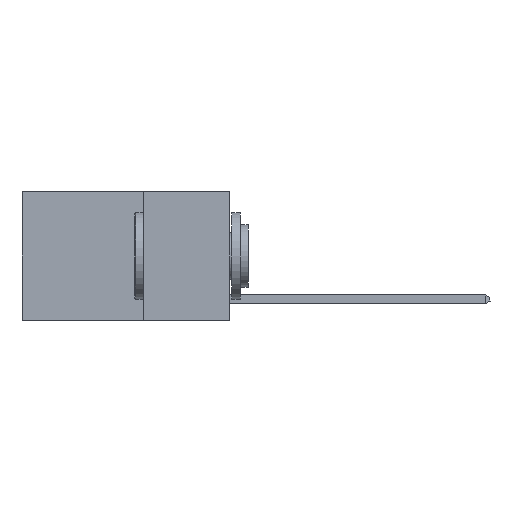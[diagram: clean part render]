
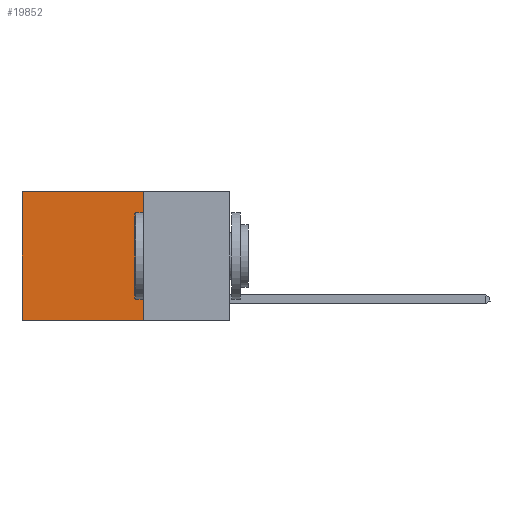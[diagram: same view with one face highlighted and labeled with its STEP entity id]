
A CAD part, left-side view. The second image highlights one B-rep face of the part: STEP entity #19852.
In plain terms, the highlighted planar face has unit normal (-1, 0, 0).
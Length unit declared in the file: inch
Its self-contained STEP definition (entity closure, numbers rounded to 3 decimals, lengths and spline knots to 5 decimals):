
#639 = AXIS2_PLACEMENT_3D ( 'NONE', #8546, #20052, #8620 ) ;
#913 = DIRECTION ( 'NONE',  ( 0., 0., -1. ) ) ;
#1865 = LINE ( 'NONE', #15309, #2870 ) ;
#2128 = EDGE_LOOP ( 'NONE', ( #5943, #13772, #2980, #7257 ) ) ;
#2133 = CARTESIAN_POINT ( 'NONE',  ( 0.2625, 0.25, 0. ) ) ;
#2255 = PLANE ( 'NONE',  #639 ) ;
#2349 = CARTESIAN_POINT ( 'NONE',  ( 0.2625, 0.25, -0.37 ) ) ;
#2870 = VECTOR ( 'NONE', #913, 39.37008 ) ;
#2980 = ORIENTED_EDGE ( 'NONE', *, *, #17382, .F. ) ;
#3601 = CARTESIAN_POINT ( 'NONE',  ( 0.2625, 0.25, -0.37 ) ) ;
#5098 = VECTOR ( 'NONE', #18875, 39.37008 ) ;
#5135 = VERTEX_POINT ( 'NONE', #18044 ) ;
#5290 = VECTOR ( 'NONE', #15388, 39.37008 ) ;
#5943 = ORIENTED_EDGE ( 'NONE', *, *, #15808, .T. ) ;
#6540 = CARTESIAN_POINT ( 'NONE',  ( 0.2625, 0.25, 0. ) ) ;
#7257 = ORIENTED_EDGE ( 'NONE', *, *, #16934, .T. ) ;
#8546 = CARTESIAN_POINT ( 'NONE',  ( 0.2625, 0.25, 0. ) ) ;
#8620 = DIRECTION ( 'NONE',  ( 0., 0., -1. ) ) ;
#8646 = VERTEX_POINT ( 'NONE', #2349 ) ;
#9038 = LINE ( 'NONE', #20776, #18311 ) ;
#9312 = DIRECTION ( 'NONE',  ( 0., 1., 0. ) ) ;
#9732 = LINE ( 'NONE', #3601, #5290 ) ;
#11012 = FACE_OUTER_BOUND ( 'NONE', #2128, .T. ) ;
#11340 = CARTESIAN_POINT ( 'NONE',  ( 0.2625, 0.6, -0.37 ) ) ;
#13772 = ORIENTED_EDGE ( 'NONE', *, *, #19311, .F. ) ;
#15309 = CARTESIAN_POINT ( 'NONE',  ( 0.2625, 0.6, 0. ) ) ;
#15388 = DIRECTION ( 'NONE',  ( 0., 1., 0. ) ) ;
#15808 = EDGE_CURVE ( 'NONE', #5135, #16032, #1865, .T. ) ;
#16032 = VERTEX_POINT ( 'NONE', #11340 ) ;
#16049 = VERTEX_POINT ( 'NONE', #6540 ) ;
#16934 = EDGE_CURVE ( 'NONE', #16049, #5135, #9038, .T. ) ;
#17382 = EDGE_CURVE ( 'NONE', #16049, #8646, #20603, .T. ) ;
#18044 = CARTESIAN_POINT ( 'NONE',  ( 0.2625, 0.6, 0. ) ) ;
#18311 = VECTOR ( 'NONE', #9312, 39.37008 ) ;
#18875 = DIRECTION ( 'NONE',  ( 0., 0., -1. ) ) ;
#19311 = EDGE_CURVE ( 'NONE', #8646, #16032, #9732, .T. ) ;
#19852 = ADVANCED_FACE ( 'NONE', ( #11012 ), #2255, .F. ) ;
#20052 = DIRECTION ( 'NONE',  ( 1., 0., 0. ) ) ;
#20603 = LINE ( 'NONE', #2133, #5098 ) ;
#20776 = CARTESIAN_POINT ( 'NONE',  ( 0.2625, 0.25, 0. ) ) ;
